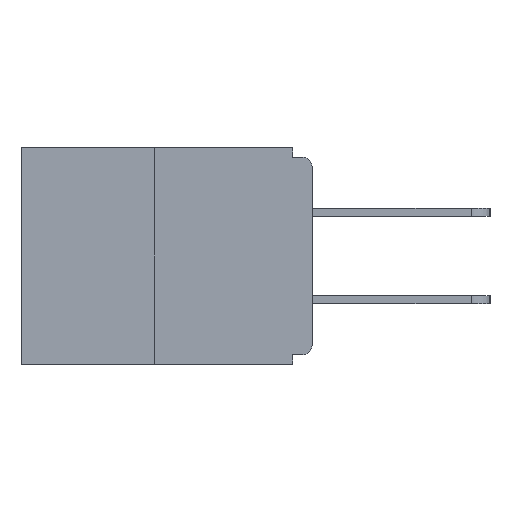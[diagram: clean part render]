
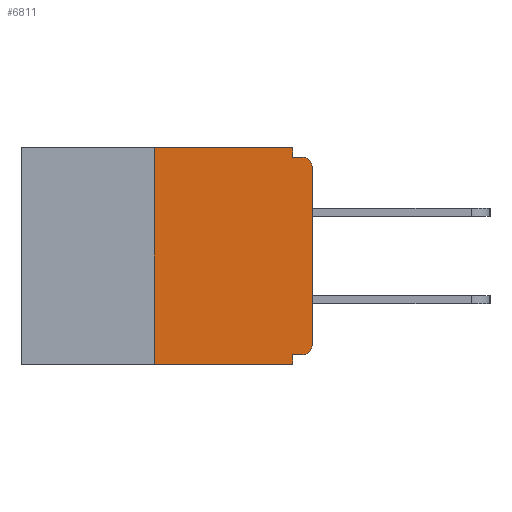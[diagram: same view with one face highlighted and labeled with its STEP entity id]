
A CAD part, left-side view. The second image highlights one B-rep face of the part: STEP entity #6811.
In plain terms, the highlighted planar face has unit normal (-1, 0, 0).
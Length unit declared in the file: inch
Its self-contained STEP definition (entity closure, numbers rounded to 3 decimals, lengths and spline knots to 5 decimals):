
#92 = EDGE_CURVE ( 'NONE', #20090, #28655, #18410, .T. ) ;
#781 = CARTESIAN_POINT ( 'NONE',  ( 0., 0.25, 0. ) ) ;
#1144 = CARTESIAN_POINT ( 'NONE',  ( 0., 0.46, 0. ) ) ;
#1632 = CARTESIAN_POINT ( 'NONE',  ( 0., 0.25, 0. ) ) ;
#1904 = EDGE_LOOP ( 'NONE', ( #20458, #20701, #18657, #23156, #29078, #4926, #4308, #19766, #25994, #24932 ) ) ;
#1968 = DIRECTION ( 'NONE',  ( -1., 0., 0. ) ) ;
#2168 = LINE ( 'NONE', #10055, #25730 ) ;
#2688 = CARTESIAN_POINT ( 'NONE',  ( 0., 0.015, -0.328 ) ) ;
#3124 = EDGE_CURVE ( 'NONE', #29045, #28655, #8655, .T. ) ;
#3489 = LINE ( 'NONE', #781, #11026 ) ;
#4088 = DIRECTION ( 'NONE',  ( 0., -1., 0. ) ) ;
#4308 = ORIENTED_EDGE ( 'NONE', *, *, #26188, .T. ) ;
#4926 = ORIENTED_EDGE ( 'NONE', *, *, #8146, .T. ) ;
#5394 = VERTEX_POINT ( 'NONE', #7708 ) ;
#5563 = DIRECTION ( 'NONE',  ( 0., 0., 1. ) ) ;
#5578 = DIRECTION ( 'NONE',  ( 0., 0., -1. ) ) ;
#5643 = FACE_OUTER_BOUND ( 'NONE', #1904, .T. ) ;
#5825 = DIRECTION ( 'NONE',  ( 0., -1., 0. ) ) ;
#6320 = VECTOR ( 'NONE', #5578, 39.37008 ) ;
#6811 = ADVANCED_FACE ( 'NONE', ( #5643 ), #28495, .F. ) ;
#6872 = CARTESIAN_POINT ( 'NONE',  ( 0., 0.031, -0.328 ) ) ;
#6874 = CARTESIAN_POINT ( 'NONE',  ( 0., 0.46, 0. ) ) ;
#7385 = VECTOR ( 'NONE', #22927, 39.37008 ) ;
#7708 = CARTESIAN_POINT ( 'NONE',  ( 0., 0.031, -0.343 ) ) ;
#7743 = EDGE_CURVE ( 'NONE', #9640, #7805, #25223, .T. ) ;
#7805 = VERTEX_POINT ( 'NONE', #6872 ) ;
#8146 = EDGE_CURVE ( 'NONE', #9640, #11778, #16263, .T. ) ;
#8655 = LINE ( 'NONE', #28754, #21490 ) ;
#9009 = EDGE_CURVE ( 'NONE', #16041, #5394, #17675, .T. ) ;
#9159 = LINE ( 'NONE', #23768, #6320 ) ;
#9640 = VERTEX_POINT ( 'NONE', #2688 ) ;
#9682 = CARTESIAN_POINT ( 'NONE',  ( 0., 0.031, 0. ) ) ;
#10055 = CARTESIAN_POINT ( 'NONE',  ( 0., 0., 0. ) ) ;
#10795 = LINE ( 'NONE', #6874, #17546 ) ;
#11026 = VECTOR ( 'NONE', #20989, 39.37008 ) ;
#11628 = EDGE_CURVE ( 'NONE', #23369, #14149, #10795, .T. ) ;
#11778 = VERTEX_POINT ( 'NONE', #24848 ) ;
#11903 = CARTESIAN_POINT ( 'NONE',  ( 0., 0.031, -0.343 ) ) ;
#12354 = CARTESIAN_POINT ( 'NONE',  ( 0., 0.25, -0.343 ) ) ;
#13485 = LINE ( 'NONE', #11903, #15632 ) ;
#13626 = DIRECTION ( 'NONE',  ( -1., 0., 0. ) ) ;
#14149 = VERTEX_POINT ( 'NONE', #9682 ) ;
#14203 = EDGE_CURVE ( 'NONE', #14149, #29045, #9159, .T. ) ;
#15268 = AXIS2_PLACEMENT_3D ( 'NONE', #20617, #13626, #29478 ) ;
#15588 = AXIS2_PLACEMENT_3D ( 'NONE', #15644, #1968, #17923 ) ;
#15632 = VECTOR ( 'NONE', #27944, 39.37008 ) ;
#15644 = CARTESIAN_POINT ( 'NONE',  ( 0., 0.015, -0.03 ) ) ;
#15952 = CARTESIAN_POINT ( 'NONE',  ( 0., 0.015, -0.015 ) ) ;
#16041 = VERTEX_POINT ( 'NONE', #12354 ) ;
#16263 = CIRCLE ( 'NONE', #15268, 0.015 ) ;
#17546 = VECTOR ( 'NONE', #22836, 39.37008 ) ;
#17675 = LINE ( 'NONE', #19109, #29114 ) ;
#17748 = EDGE_CURVE ( 'NONE', #16041, #23369, #3489, .T. ) ;
#17923 = DIRECTION ( 'NONE',  ( 0., 0., -1. ) ) ;
#18410 = CIRCLE ( 'NONE', #15588, 0.015 ) ;
#18657 = ORIENTED_EDGE ( 'NONE', *, *, #9009, .T. ) ;
#19109 = CARTESIAN_POINT ( 'NONE',  ( 0., 0.46, -0.343 ) ) ;
#19170 = EDGE_CURVE ( 'NONE', #7805, #5394, #13485, .T. ) ;
#19766 = ORIENTED_EDGE ( 'NONE', *, *, #92, .T. ) ;
#20090 = VERTEX_POINT ( 'NONE', #26878 ) ;
#20458 = ORIENTED_EDGE ( 'NONE', *, *, #11628, .F. ) ;
#20617 = CARTESIAN_POINT ( 'NONE',  ( 0., 0.015, -0.313 ) ) ;
#20701 = ORIENTED_EDGE ( 'NONE', *, *, #17748, .F. ) ;
#20989 = DIRECTION ( 'NONE',  ( 0., 0., 1. ) ) ;
#21490 = VECTOR ( 'NONE', #4088, 39.37008 ) ;
#21933 = DIRECTION ( 'NONE',  ( 0., 0., -1. ) ) ;
#21946 = CARTESIAN_POINT ( 'NONE',  ( 0., 0.031, -0.015 ) ) ;
#22836 = DIRECTION ( 'NONE',  ( 0., -1., 0. ) ) ;
#22927 = DIRECTION ( 'NONE',  ( 0., 1., 0. ) ) ;
#23156 = ORIENTED_EDGE ( 'NONE', *, *, #19170, .F. ) ;
#23369 = VERTEX_POINT ( 'NONE', #1632 ) ;
#23768 = CARTESIAN_POINT ( 'NONE',  ( 0., 0.031, 0. ) ) ;
#24848 = CARTESIAN_POINT ( 'NONE',  ( 0., 0., -0.313 ) ) ;
#24932 = ORIENTED_EDGE ( 'NONE', *, *, #14203, .F. ) ;
#25223 = LINE ( 'NONE', #27236, #7385 ) ;
#25730 = VECTOR ( 'NONE', #5563, 39.37008 ) ;
#25731 = AXIS2_PLACEMENT_3D ( 'NONE', #1144, #26608, #21933 ) ;
#25994 = ORIENTED_EDGE ( 'NONE', *, *, #3124, .F. ) ;
#26188 = EDGE_CURVE ( 'NONE', #11778, #20090, #2168, .T. ) ;
#26608 = DIRECTION ( 'NONE',  ( 1., 0., 0. ) ) ;
#26878 = CARTESIAN_POINT ( 'NONE',  ( 0., 0., -0.03 ) ) ;
#27236 = CARTESIAN_POINT ( 'NONE',  ( 0., 0., -0.328 ) ) ;
#27944 = DIRECTION ( 'NONE',  ( 0., 0., -1. ) ) ;
#28495 = PLANE ( 'NONE',  #25731 ) ;
#28655 = VERTEX_POINT ( 'NONE', #15952 ) ;
#28754 = CARTESIAN_POINT ( 'NONE',  ( 0., 0., -0.015 ) ) ;
#29045 = VERTEX_POINT ( 'NONE', #21946 ) ;
#29078 = ORIENTED_EDGE ( 'NONE', *, *, #7743, .F. ) ;
#29114 = VECTOR ( 'NONE', #5825, 39.37008 ) ;
#29478 = DIRECTION ( 'NONE',  ( 0., 0., -1. ) ) ;
